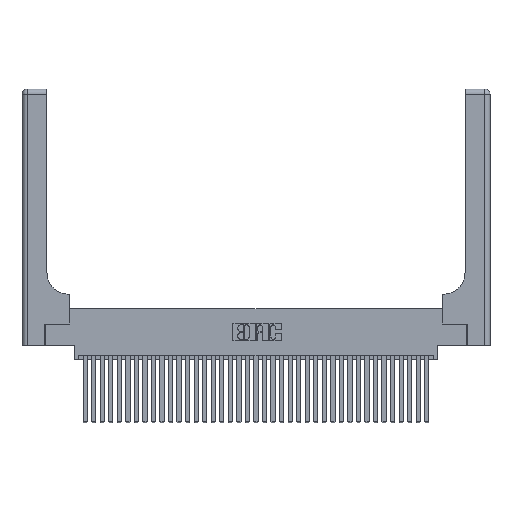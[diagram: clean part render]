
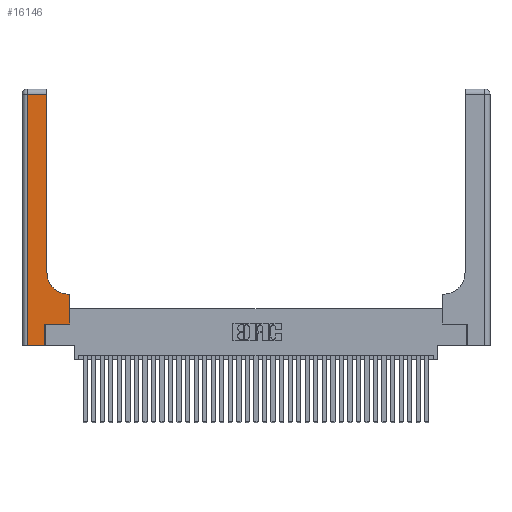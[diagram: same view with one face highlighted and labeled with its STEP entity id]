
A CAD part, top view. The second image highlights one B-rep face of the part: STEP entity #16146.
In plain terms, the highlighted planar face has unit normal (0, 0, 1).
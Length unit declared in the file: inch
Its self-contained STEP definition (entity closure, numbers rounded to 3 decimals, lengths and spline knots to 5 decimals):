
#552 = EDGE_CURVE ( 'NONE', #35543, #28570, #1838, .T. ) ;
#788 = CARTESIAN_POINT ( 'NONE',  ( 0.269, 0.25, 0.37 ) ) ;
#1110 = EDGE_LOOP ( 'NONE', ( #27959, #36400, #5269, #21941, #37393, #36442, #15195, #17042, #1835 ) ) ;
#1221 = LINE ( 'NONE', #8738, #23429 ) ;
#1474 = DIRECTION ( 'NONE',  ( -1., 0., 0. ) ) ;
#1505 = LINE ( 'NONE', #37217, #20577 ) ;
#1835 = ORIENTED_EDGE ( 'NONE', *, *, #552, .T. ) ;
#1838 = CIRCLE ( 'NONE', #33107, 0.25 ) ;
#2790 = DIRECTION ( 'NONE',  ( 0., 1., 0. ) ) ;
#3244 = VERTEX_POINT ( 'NONE', #21652 ) ;
#4121 = CARTESIAN_POINT ( 'NONE',  ( 0.06, 0., 0.37 ) ) ;
#5269 = ORIENTED_EDGE ( 'NONE', *, *, #37313, .T. ) ;
#5713 = EDGE_CURVE ( 'NONE', #29347, #36405, #1505, .T. ) ;
#6360 = DIRECTION ( 'NONE',  ( 1., 0., 0. ) ) ;
#6578 = CARTESIAN_POINT ( 'NONE',  ( 0.06, 2.94, 0.37 ) ) ;
#7825 = CARTESIAN_POINT ( 'NONE',  ( 0.269, 0., 0.37 ) ) ;
#8738 = CARTESIAN_POINT ( 'NONE',  ( 0.06, 3., 0.37 ) ) ;
#9245 = CARTESIAN_POINT ( 'NONE',  ( 0.2915, 3., 0.37 ) ) ;
#9771 = AXIS2_PLACEMENT_3D ( 'NONE', #18738, #21508, #1474 ) ;
#9887 = CARTESIAN_POINT ( 'NONE',  ( 0.5415, 0.85, 0.37 ) ) ;
#10481 = FACE_OUTER_BOUND ( 'NONE', #1110, .T. ) ;
#10685 = VECTOR ( 'NONE', #20928, 39.37008 ) ;
#10800 = EDGE_CURVE ( 'NONE', #20657, #30742, #35532, .T. ) ;
#10818 = VECTOR ( 'NONE', #33741, 39.37008 ) ;
#12380 = DIRECTION ( 'NONE',  ( -1., 0., 0. ) ) ;
#12510 = EDGE_CURVE ( 'NONE', #30742, #32933, #16700, .T. ) ;
#13095 = VECTOR ( 'NONE', #29346, 39.37008 ) ;
#14939 = CARTESIAN_POINT ( 'NONE',  ( 0.2915, 0.85, 0.37 ) ) ;
#15195 = ORIENTED_EDGE ( 'NONE', *, *, #12510, .T. ) ;
#15537 = PLANE ( 'NONE',  #9771 ) ;
#15539 = CARTESIAN_POINT ( 'NONE',  ( 0.269, 0.25, 0.37 ) ) ;
#16022 = CARTESIAN_POINT ( 'NONE',  ( 0.5415, 0.6, 0.37 ) ) ;
#16146 = ADVANCED_FACE ( 'NONE', ( #10481 ), #15537, .F. ) ;
#16219 = CARTESIAN_POINT ( 'NONE',  ( 0., 2.94, 0.37 ) ) ;
#16700 = LINE ( 'NONE', #17138, #36091 ) ;
#17042 = ORIENTED_EDGE ( 'NONE', *, *, #18673, .T. ) ;
#17138 = CARTESIAN_POINT ( 'NONE',  ( 0.5585, 0.25, 0.37 ) ) ;
#17394 = CARTESIAN_POINT ( 'NONE',  ( 0.269, 0., 0.37 ) ) ;
#17751 = DIRECTION ( 'NONE',  ( 0., -1., 0. ) ) ;
#18416 = LINE ( 'NONE', #9245, #10685 ) ;
#18563 = LINE ( 'NONE', #16219, #10818 ) ;
#18607 = LINE ( 'NONE', #17394, #13095 ) ;
#18673 = EDGE_CURVE ( 'NONE', #32933, #35543, #37241, .T. ) ;
#18738 = CARTESIAN_POINT ( 'NONE',  ( 0., 3., 0.37 ) ) ;
#20577 = VECTOR ( 'NONE', #6360, 39.37008 ) ;
#20657 = VERTEX_POINT ( 'NONE', #15539 ) ;
#20928 = DIRECTION ( 'NONE',  ( 0., 1., 0. ) ) ;
#21508 = DIRECTION ( 'NONE',  ( 0., 0., -1. ) ) ;
#21652 = CARTESIAN_POINT ( 'NONE',  ( 0.2915, 2.94, 0.37 ) ) ;
#21941 = ORIENTED_EDGE ( 'NONE', *, *, #5713, .T. ) ;
#23429 = VECTOR ( 'NONE', #17751, 39.37008 ) ;
#23833 = DIRECTION ( 'NONE',  ( 1., 0., 0. ) ) ;
#25035 = VECTOR ( 'NONE', #12380, 39.37008 ) ;
#27959 = ORIENTED_EDGE ( 'NONE', *, *, #30443, .T. ) ;
#28570 = VERTEX_POINT ( 'NONE', #14939 ) ;
#29346 = DIRECTION ( 'NONE',  ( 0., 1., 0. ) ) ;
#29347 = VERTEX_POINT ( 'NONE', #4121 ) ;
#29548 = CARTESIAN_POINT ( 'NONE',  ( 0.2915, 0.6, 0.37 ) ) ;
#29859 = DIRECTION ( 'NONE',  ( 0., 0., -1. ) ) ;
#30443 = EDGE_CURVE ( 'NONE', #28570, #3244, #18416, .T. ) ;
#30515 = VERTEX_POINT ( 'NONE', #6578 ) ;
#30742 = VERTEX_POINT ( 'NONE', #34071 ) ;
#31900 = VECTOR ( 'NONE', #23833, 39.37008 ) ;
#32933 = VERTEX_POINT ( 'NONE', #34822 ) ;
#33107 = AXIS2_PLACEMENT_3D ( 'NONE', #9887, #29859, #35659 ) ;
#33741 = DIRECTION ( 'NONE',  ( -1., 0., 0. ) ) ;
#34071 = CARTESIAN_POINT ( 'NONE',  ( 0.5585, 0.25, 0.37 ) ) ;
#34822 = CARTESIAN_POINT ( 'NONE',  ( 0.5585, 0.6, 0.37 ) ) ;
#35532 = LINE ( 'NONE', #788, #31900 ) ;
#35543 = VERTEX_POINT ( 'NONE', #16022 ) ;
#35659 = DIRECTION ( 'NONE',  ( 1., 0., 0. ) ) ;
#35947 = EDGE_CURVE ( 'NONE', #36405, #20657, #18607, .T. ) ;
#36091 = VECTOR ( 'NONE', #2790, 39.37008 ) ;
#36261 = EDGE_CURVE ( 'NONE', #3244, #30515, #18563, .T. ) ;
#36400 = ORIENTED_EDGE ( 'NONE', *, *, #36261, .T. ) ;
#36405 = VERTEX_POINT ( 'NONE', #7825 ) ;
#36442 = ORIENTED_EDGE ( 'NONE', *, *, #10800, .T. ) ;
#37217 = CARTESIAN_POINT ( 'NONE',  ( 0., 0., 0.37 ) ) ;
#37241 = LINE ( 'NONE', #29548, #25035 ) ;
#37313 = EDGE_CURVE ( 'NONE', #30515, #29347, #1221, .T. ) ;
#37393 = ORIENTED_EDGE ( 'NONE', *, *, #35947, .T. ) ;
